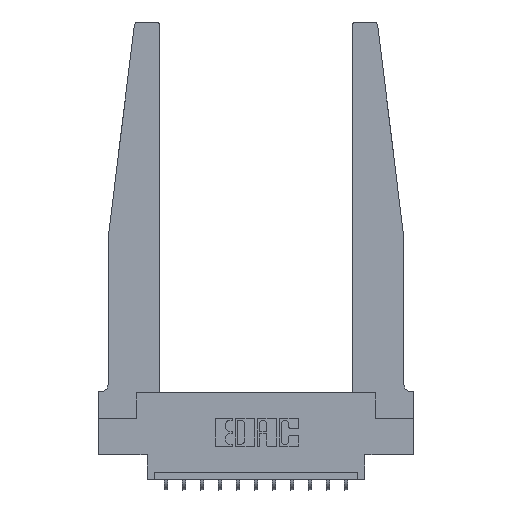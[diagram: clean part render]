
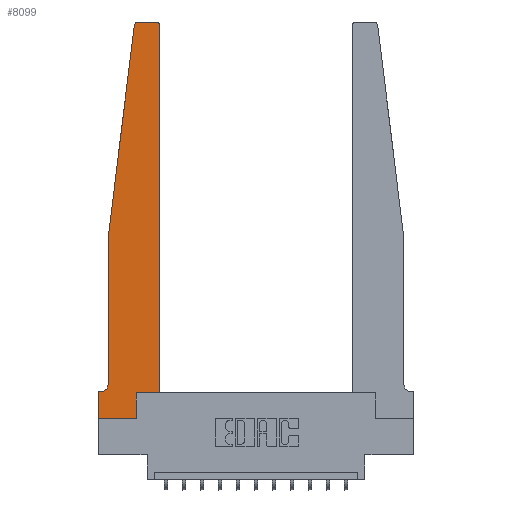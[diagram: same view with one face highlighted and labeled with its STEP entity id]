
A CAD part, top view. The second image highlights one B-rep face of the part: STEP entity #8099.
In plain terms, the highlighted planar face has unit normal (0, 0, 1).
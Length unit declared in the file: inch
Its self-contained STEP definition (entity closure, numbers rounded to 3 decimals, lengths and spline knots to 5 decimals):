
#79 = VECTOR ( 'NONE', #15578, 39.37008 ) ;
#84 = CARTESIAN_POINT ( 'NONE',  ( 0.2605, 0., 0.37 ) ) ;
#150 = ORIENTED_EDGE ( 'NONE', *, *, #7797, .T. ) ;
#489 = CARTESIAN_POINT ( 'NONE',  ( 0.015, 0.2375, 0.37 ) ) ;
#584 = VECTOR ( 'NONE', #4258, 39.37008 ) ;
#836 = LINE ( 'NONE', #7113, #7449 ) ;
#1017 = CARTESIAN_POINT ( 'NONE',  ( 0.065, 0.2375, 0.37 ) ) ;
#1059 = CARTESIAN_POINT ( 'NONE',  ( 0.2605, 0.18, 0.37 ) ) ;
#1203 = ORIENTED_EDGE ( 'NONE', *, *, #2611, .T. ) ;
#1421 = LINE ( 'NONE', #15359, #4053 ) ;
#1497 = EDGE_CURVE ( 'NONE', #12397, #6041, #12420, .T. ) ;
#1512 = CIRCLE ( 'NONE', #16364, 0.05 ) ;
#1733 = AXIS2_PLACEMENT_3D ( 'NONE', #13894, #11333, #10327 ) ;
#1858 = DIRECTION ( 'NONE',  ( 0., -1., 0. ) ) ;
#2212 = CARTESIAN_POINT ( 'NONE',  ( 0.395, 2.75, 0.37 ) ) ;
#2215 = CARTESIAN_POINT ( 'NONE',  ( 0.425, 2.72, 0.37 ) ) ;
#2245 = CIRCLE ( 'NONE', #1733, 0.03 ) ;
#2611 = EDGE_CURVE ( 'NONE', #6041, #5670, #836, .T. ) ;
#2727 = AXIS2_PLACEMENT_3D ( 'NONE', #10407, #6396, #10156 ) ;
#2857 = DIRECTION ( 'NONE',  ( -1., 0., 0. ) ) ;
#3008 = CARTESIAN_POINT ( 'NONE',  ( 0., 0., 0.37 ) ) ;
#3059 = LINE ( 'NONE', #4313, #3317 ) ;
#3108 = ORIENTED_EDGE ( 'NONE', *, *, #6291, .T. ) ;
#3317 = VECTOR ( 'NONE', #4387, 39.37008 ) ;
#3573 = VECTOR ( 'NONE', #4503, 39.37008 ) ;
#3620 = EDGE_CURVE ( 'NONE', #8786, #13743, #2245, .T. ) ;
#3832 = CARTESIAN_POINT ( 'NONE',  ( 0.24675, 2.72367, 0.37 ) ) ;
#3922 = FACE_OUTER_BOUND ( 'NONE', #11483, .T. ) ;
#3972 = VERTEX_POINT ( 'NONE', #1017 ) ;
#3985 = ORIENTED_EDGE ( 'NONE', *, *, #3620, .T. ) ;
#3988 = DIRECTION ( 'NONE',  ( 0., 1., 0. ) ) ;
#4052 = CARTESIAN_POINT ( 'NONE',  ( 0.065, 1.25, 0.37 ) ) ;
#4053 = VECTOR ( 'NONE', #11634, 39.37008 ) ;
#4129 = CARTESIAN_POINT ( 'NONE',  ( 0.065, 1.25, 0.37 ) ) ;
#4258 = DIRECTION ( 'NONE',  ( 1., 0., 0. ) ) ;
#4313 = CARTESIAN_POINT ( 'NONE',  ( 0.25, 2.75, 0.37 ) ) ;
#4387 = DIRECTION ( 'NONE',  ( -1., 0., 0. ) ) ;
#4503 = DIRECTION ( 'NONE',  ( -0.122, -0.992, 0. ) ) ;
#4630 = DIRECTION ( 'NONE',  ( 1., 0., 0. ) ) ;
#5317 = EDGE_CURVE ( 'NONE', #5670, #8786, #11406, .T. ) ;
#5490 = CARTESIAN_POINT ( 'NONE',  ( 0.27653, 2.72, 0.37 ) ) ;
#5594 = CARTESIAN_POINT ( 'NONE',  ( 0., 0., 0.37 ) ) ;
#5670 = VERTEX_POINT ( 'NONE', #14771 ) ;
#6041 = VERTEX_POINT ( 'NONE', #8278 ) ;
#6098 = DIRECTION ( 'NONE',  ( 0., 1., 0. ) ) ;
#6291 = EDGE_CURVE ( 'NONE', #3972, #6553, #1512, .T. ) ;
#6325 = VERTEX_POINT ( 'NONE', #12235 ) ;
#6396 = DIRECTION ( 'NONE',  ( 0., 0., 1. ) ) ;
#6445 = ORIENTED_EDGE ( 'NONE', *, *, #1497, .T. ) ;
#6553 = VERTEX_POINT ( 'NONE', #16283 ) ;
#6960 = CARTESIAN_POINT ( 'NONE',  ( 0.27653, 2.75, 0.37 ) ) ;
#7113 = CARTESIAN_POINT ( 'NONE',  ( 0.425, 0.18, 0.37 ) ) ;
#7449 = VECTOR ( 'NONE', #4630, 39.37008 ) ;
#7797 = EDGE_CURVE ( 'NONE', #6325, #12967, #14419, .T. ) ;
#7881 = LINE ( 'NONE', #4052, #3573 ) ;
#8099 = ADVANCED_FACE ( 'NONE', ( #3922 ), #9064, .T. ) ;
#8220 = VERTEX_POINT ( 'NONE', #3832 ) ;
#8278 = CARTESIAN_POINT ( 'NONE',  ( 0.2605, 0.18, 0.37 ) ) ;
#8786 = VERTEX_POINT ( 'NONE', #2215 ) ;
#8969 = EDGE_CURVE ( 'NONE', #8220, #10899, #7881, .T. ) ;
#8989 = VECTOR ( 'NONE', #1858, 39.37008 ) ;
#9064 = PLANE ( 'NONE',  #2727 ) ;
#9188 = LINE ( 'NONE', #4129, #79 ) ;
#9469 = VECTOR ( 'NONE', #3988, 39.37008 ) ;
#9542 = CARTESIAN_POINT ( 'NONE',  ( 0., 0., 0.37 ) ) ;
#9825 = EDGE_CURVE ( 'NONE', #13743, #11737, #3059, .T. ) ;
#9899 = VECTOR ( 'NONE', #6098, 39.37008 ) ;
#10156 = DIRECTION ( 'NONE',  ( 1., 0., 0. ) ) ;
#10327 = DIRECTION ( 'NONE',  ( 1., 0., 0. ) ) ;
#10354 = ORIENTED_EDGE ( 'NONE', *, *, #14973, .T. ) ;
#10379 = EDGE_CURVE ( 'NONE', #11737, #8220, #13269, .T. ) ;
#10407 = CARTESIAN_POINT ( 'NONE',  ( 0., 0.1875, 0.37 ) ) ;
#10670 = LINE ( 'NONE', #3008, #584 ) ;
#10899 = VERTEX_POINT ( 'NONE', #15671 ) ;
#11191 = EDGE_CURVE ( 'NONE', #12967, #12397, #10670, .T. ) ;
#11333 = DIRECTION ( 'NONE',  ( 0., 0., 1. ) ) ;
#11406 = LINE ( 'NONE', #13879, #9469 ) ;
#11483 = EDGE_LOOP ( 'NONE', ( #15888, #14146, #15971, #15622, #3108, #10354, #150, #12007, #6445, #1203, #16192, #3985 ) ) ;
#11634 = DIRECTION ( 'NONE',  ( -1., 0., 0. ) ) ;
#11737 = VERTEX_POINT ( 'NONE', #6960 ) ;
#11919 = DIRECTION ( 'NONE',  ( 0., 0., -1. ) ) ;
#12007 = ORIENTED_EDGE ( 'NONE', *, *, #11191, .T. ) ;
#12235 = CARTESIAN_POINT ( 'NONE',  ( 0., 0.1875, 0.37 ) ) ;
#12397 = VERTEX_POINT ( 'NONE', #84 ) ;
#12420 = LINE ( 'NONE', #1059, #9899 ) ;
#12967 = VERTEX_POINT ( 'NONE', #9542 ) ;
#13269 = CIRCLE ( 'NONE', #15136, 0.03 ) ;
#13743 = VERTEX_POINT ( 'NONE', #2212 ) ;
#13789 = EDGE_CURVE ( 'NONE', #10899, #3972, #9188, .T. ) ;
#13879 = CARTESIAN_POINT ( 'NONE',  ( 0.425, 0.18, 0.37 ) ) ;
#13894 = CARTESIAN_POINT ( 'NONE',  ( 0.395, 2.72, 0.37 ) ) ;
#14146 = ORIENTED_EDGE ( 'NONE', *, *, #10379, .T. ) ;
#14303 = DIRECTION ( 'NONE',  ( 0., 0., 1. ) ) ;
#14419 = LINE ( 'NONE', #5594, #8989 ) ;
#14771 = CARTESIAN_POINT ( 'NONE',  ( 0.425, 0.18, 0.37 ) ) ;
#14973 = EDGE_CURVE ( 'NONE', #6553, #6325, #1421, .T. ) ;
#15136 = AXIS2_PLACEMENT_3D ( 'NONE', #5490, #14303, #15536 ) ;
#15359 = CARTESIAN_POINT ( 'NONE',  ( 0.065, 0.1875, 0.37 ) ) ;
#15536 = DIRECTION ( 'NONE',  ( 1., 0., 0. ) ) ;
#15578 = DIRECTION ( 'NONE',  ( 0., -1., 0. ) ) ;
#15622 = ORIENTED_EDGE ( 'NONE', *, *, #13789, .T. ) ;
#15671 = CARTESIAN_POINT ( 'NONE',  ( 0.065, 1.25, 0.37 ) ) ;
#15888 = ORIENTED_EDGE ( 'NONE', *, *, #9825, .T. ) ;
#15971 = ORIENTED_EDGE ( 'NONE', *, *, #8969, .T. ) ;
#16192 = ORIENTED_EDGE ( 'NONE', *, *, #5317, .T. ) ;
#16283 = CARTESIAN_POINT ( 'NONE',  ( 0.015, 0.1875, 0.37 ) ) ;
#16364 = AXIS2_PLACEMENT_3D ( 'NONE', #489, #11919, #2857 ) ;
